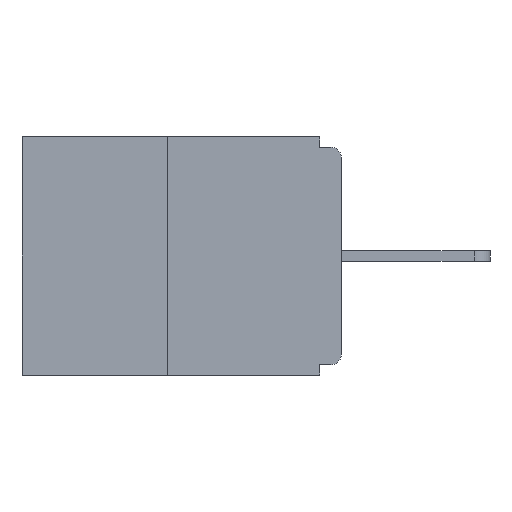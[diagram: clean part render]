
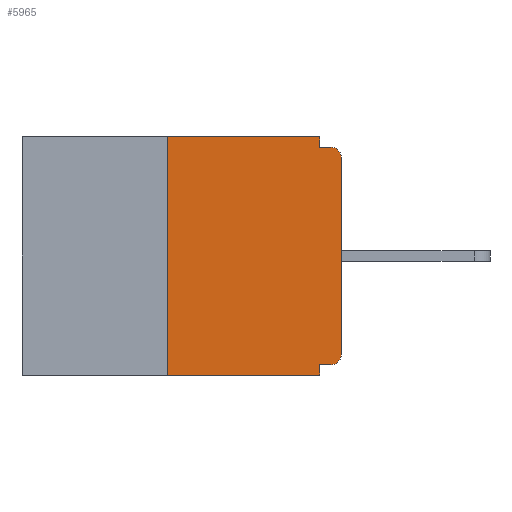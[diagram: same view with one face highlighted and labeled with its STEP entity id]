
A CAD part, left-side view. The second image highlights one B-rep face of the part: STEP entity #5965.
In plain terms, the highlighted planar face has unit normal (-1, 0, 0).
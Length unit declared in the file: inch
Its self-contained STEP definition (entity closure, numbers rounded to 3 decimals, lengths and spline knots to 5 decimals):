
#15 = FACE_OUTER_BOUND ( 'NONE', #3957, .T. ) ;
#24 = VECTOR ( 'NONE', #8827, 39.37008 ) ;
#88 = CARTESIAN_POINT ( 'NONE',  ( 0., 0.031, -0.328 ) ) ;
#224 = CARTESIAN_POINT ( 'NONE',  ( 0., 0.015, -0.015 ) ) ;
#240 = EDGE_CURVE ( 'NONE', #2160, #3615, #2670, .T. ) ;
#242 = CARTESIAN_POINT ( 'NONE',  ( 0., 0., -0.015 ) ) ;
#258 = ORIENTED_EDGE ( 'NONE', *, *, #5113, .F. ) ;
#711 = ORIENTED_EDGE ( 'NONE', *, *, #9051, .T. ) ;
#790 = CARTESIAN_POINT ( 'NONE',  ( 0., 0., 0. ) ) ;
#897 = DIRECTION ( 'NONE',  ( 0., 0., -1. ) ) ;
#956 = CARTESIAN_POINT ( 'NONE',  ( 0., 0.031, -0.343 ) ) ;
#991 = CIRCLE ( 'NONE', #2455, 0.015 ) ;
#1017 = CARTESIAN_POINT ( 'NONE',  ( 0., 0.015, -0.328 ) ) ;
#1072 = DIRECTION ( 'NONE',  ( 0., 0., -1. ) ) ;
#1130 = CARTESIAN_POINT ( 'NONE',  ( 0., 0.031, 0. ) ) ;
#1375 = DIRECTION ( 'NONE',  ( 0., 0., -1. ) ) ;
#1669 = EDGE_CURVE ( 'NONE', #9437, #6327, #5444, .T. ) ;
#1677 = VECTOR ( 'NONE', #5223, 39.37008 ) ;
#1685 = EDGE_CURVE ( 'NONE', #8220, #3615, #1797, .T. ) ;
#1746 = ORIENTED_EDGE ( 'NONE', *, *, #1669, .F. ) ;
#1797 = CIRCLE ( 'NONE', #9890, 0.015 ) ;
#1860 = DIRECTION ( 'NONE',  ( 0., 0., -1. ) ) ;
#1980 = PLANE ( 'NONE',  #7772 ) ;
#1983 = DIRECTION ( 'NONE',  ( -1., 0., 0. ) ) ;
#2160 = VERTEX_POINT ( 'NONE', #3471 ) ;
#2416 = LINE ( 'NONE', #5972, #1677 ) ;
#2455 = AXIS2_PLACEMENT_3D ( 'NONE', #7672, #6972, #1375 ) ;
#2557 = CARTESIAN_POINT ( 'NONE',  ( 0., 0.25, 0. ) ) ;
#2670 = LINE ( 'NONE', #242, #6391 ) ;
#2737 = LINE ( 'NONE', #3610, #24 ) ;
#2975 = VECTOR ( 'NONE', #3316, 39.37008 ) ;
#3213 = ORIENTED_EDGE ( 'NONE', *, *, #5868, .T. ) ;
#3316 = DIRECTION ( 'NONE',  ( 0., 0., 1. ) ) ;
#3371 = LINE ( 'NONE', #2557, #8526 ) ;
#3471 = CARTESIAN_POINT ( 'NONE',  ( 0., 0.031, -0.015 ) ) ;
#3539 = CARTESIAN_POINT ( 'NONE',  ( 0., 0.46, 0. ) ) ;
#3610 = CARTESIAN_POINT ( 'NONE',  ( 0., 0., -0.328 ) ) ;
#3615 = VERTEX_POINT ( 'NONE', #224 ) ;
#3661 = CARTESIAN_POINT ( 'NONE',  ( 0., 0.015, -0.03 ) ) ;
#3695 = VERTEX_POINT ( 'NONE', #9314 ) ;
#3957 = EDGE_LOOP ( 'NONE', ( #10463, #4593, #711, #1746, #10931, #3213, #10007, #8910, #7483, #258 ) ) ;
#4326 = CARTESIAN_POINT ( 'NONE',  ( 0., 0.031, -0.343 ) ) ;
#4400 = DIRECTION ( 'NONE',  ( 0., 0., -1. ) ) ;
#4460 = VERTEX_POINT ( 'NONE', #6396 ) ;
#4593 = ORIENTED_EDGE ( 'NONE', *, *, #7580, .F. ) ;
#5113 = EDGE_CURVE ( 'NONE', #8853, #2160, #9166, .T. ) ;
#5223 = DIRECTION ( 'NONE',  ( 0., -1., 0. ) ) ;
#5444 = LINE ( 'NONE', #956, #7122 ) ;
#5790 = CARTESIAN_POINT ( 'NONE',  ( 0., 0.25, 0. ) ) ;
#5868 = EDGE_CURVE ( 'NONE', #7594, #3695, #991, .T. ) ;
#5965 = ADVANCED_FACE ( 'NONE', ( #15 ), #1980, .F. ) ;
#5972 = CARTESIAN_POINT ( 'NONE',  ( 0., 0.46, -0.343 ) ) ;
#6327 = VERTEX_POINT ( 'NONE', #4326 ) ;
#6391 = VECTOR ( 'NONE', #10738, 39.37008 ) ;
#6396 = CARTESIAN_POINT ( 'NONE',  ( 0., 0.25, -0.343 ) ) ;
#6805 = LINE ( 'NONE', #790, #2975 ) ;
#6855 = LINE ( 'NONE', #11158, #11263 ) ;
#6972 = DIRECTION ( 'NONE',  ( -1., 0., 0. ) ) ;
#6986 = CARTESIAN_POINT ( 'NONE',  ( 0., 0., -0.03 ) ) ;
#7032 = DIRECTION ( 'NONE',  ( 1., 0., 0. ) ) ;
#7122 = VECTOR ( 'NONE', #897, 39.37008 ) ;
#7483 = ORIENTED_EDGE ( 'NONE', *, *, #240, .F. ) ;
#7580 = EDGE_CURVE ( 'NONE', #4460, #10409, #3371, .T. ) ;
#7594 = VERTEX_POINT ( 'NONE', #1017 ) ;
#7672 = CARTESIAN_POINT ( 'NONE',  ( 0., 0.015, -0.313 ) ) ;
#7720 = DIRECTION ( 'NONE',  ( 0., -1., 0. ) ) ;
#7772 = AXIS2_PLACEMENT_3D ( 'NONE', #3539, #7032, #1860 ) ;
#8220 = VERTEX_POINT ( 'NONE', #6986 ) ;
#8336 = CARTESIAN_POINT ( 'NONE',  ( 0., 0.031, 0. ) ) ;
#8526 = VECTOR ( 'NONE', #10453, 39.37008 ) ;
#8827 = DIRECTION ( 'NONE',  ( 0., 1., 0. ) ) ;
#8853 = VERTEX_POINT ( 'NONE', #8336 ) ;
#8910 = ORIENTED_EDGE ( 'NONE', *, *, #1685, .T. ) ;
#9051 = EDGE_CURVE ( 'NONE', #4460, #6327, #2416, .T. ) ;
#9166 = LINE ( 'NONE', #1130, #10344 ) ;
#9314 = CARTESIAN_POINT ( 'NONE',  ( 0., 0., -0.313 ) ) ;
#9351 = EDGE_CURVE ( 'NONE', #3695, #8220, #6805, .T. ) ;
#9437 = VERTEX_POINT ( 'NONE', #88 ) ;
#9538 = EDGE_CURVE ( 'NONE', #7594, #9437, #2737, .T. ) ;
#9730 = EDGE_CURVE ( 'NONE', #10409, #8853, #6855, .T. ) ;
#9890 = AXIS2_PLACEMENT_3D ( 'NONE', #3661, #1983, #4400 ) ;
#10007 = ORIENTED_EDGE ( 'NONE', *, *, #9351, .T. ) ;
#10344 = VECTOR ( 'NONE', #1072, 39.37008 ) ;
#10409 = VERTEX_POINT ( 'NONE', #5790 ) ;
#10453 = DIRECTION ( 'NONE',  ( 0., 0., 1. ) ) ;
#10463 = ORIENTED_EDGE ( 'NONE', *, *, #9730, .F. ) ;
#10738 = DIRECTION ( 'NONE',  ( 0., -1., 0. ) ) ;
#10931 = ORIENTED_EDGE ( 'NONE', *, *, #9538, .F. ) ;
#11158 = CARTESIAN_POINT ( 'NONE',  ( 0., 0.46, 0. ) ) ;
#11263 = VECTOR ( 'NONE', #7720, 39.37008 ) ;
